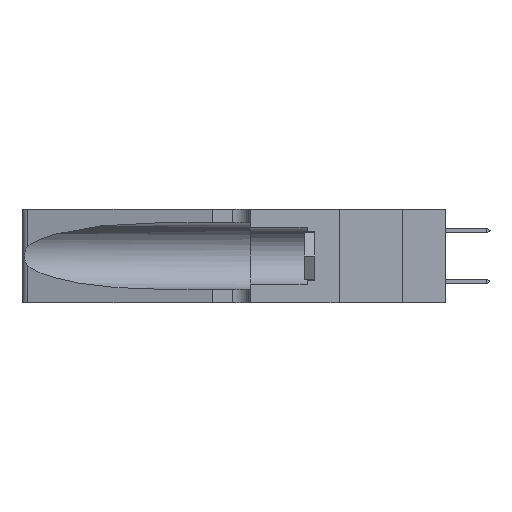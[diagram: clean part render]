
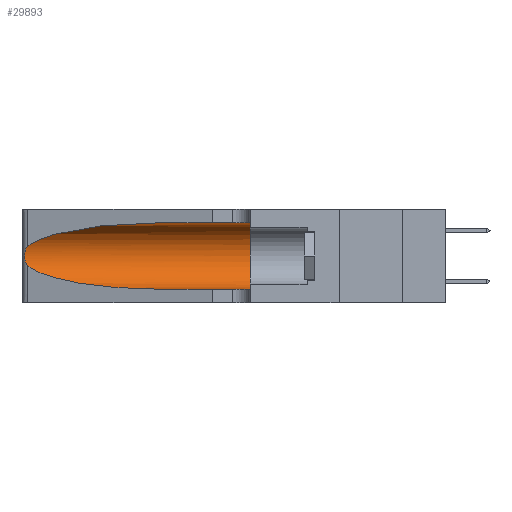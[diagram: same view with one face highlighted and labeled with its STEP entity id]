
A CAD part, left-side view. The second image highlights one B-rep face of the part: STEP entity #29893.
In plain terms, the highlighted cylindrical face has radius 3.308 mm (diameter 6.617 mm), a partial arc.
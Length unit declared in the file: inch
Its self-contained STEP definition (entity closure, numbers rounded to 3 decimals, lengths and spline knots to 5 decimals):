
#35 = DIRECTION ( 'NONE',  ( 0., -1., 0. ) ) ;
#92 = EDGE_CURVE ( 'NONE', #33186, #20749, #12099, .T. ) ;
#208 = ORIENTED_EDGE ( 'NONE', *, *, #2421, .F. ) ;
#2421 = EDGE_CURVE ( 'NONE', #32712, #20749, #4172, .T. ) ;
#4097 = DIRECTION ( 'NONE',  ( 0., -1., 0. ) ) ;
#4172 = CIRCLE ( 'NONE', #7945, 0.13025 ) ;
#4698 = VECTOR ( 'NONE', #35, 39.37008 ) ;
#5731 = EDGE_CURVE ( 'NONE', #13595, #32712, #8255, .T. ) ;
#6392 = CARTESIAN_POINT ( 'NONE',  ( 0.2373, 1.15595, 0.28018 ) ) ;
#7009 = FACE_OUTER_BOUND ( 'NONE', #9619, .T. ) ;
#7945 = AXIS2_PLACEMENT_3D ( 'NONE', #35075, #29318, #26775 ) ;
#8255 = LINE ( 'NONE', #17349, #29503 ) ;
#9052 = CARTESIAN_POINT ( 'NONE',  ( 0.25487, 1.22718, 0.22369 ) ) ;
#9436 = CARTESIAN_POINT ( 'NONE',  ( 0.1305, 1.61858, 0.185 ) ) ;
#9619 = EDGE_LOOP ( 'NONE', ( #25648, #12728, #35269, #34391, #208, #23383 ) ) ;
#9838 = EDGE_CURVE ( 'NONE', #16132, #19628, #12840, .T. ) ;
#10310 = CARTESIAN_POINT ( 'NONE',  ( 0.1305, 0.72297, 0.05475 ) ) ;
#10781 = CARTESIAN_POINT ( 'NONE',  ( 0.25639, 1.23184, 0.21858 ) ) ;
#10813 =( BOUNDED_CURVE ( )  B_SPLINE_CURVE ( 3, ( #31045, #31161, #6392, #9052 ),
 .UNSPECIFIED., .F., .F. ) 
 B_SPLINE_CURVE_WITH_KNOTS ( ( 4, 4 ),
 ( 1.5708, 2.84003 ),
 .UNSPECIFIED. ) 
 CURVE ( )  GEOMETRIC_REPRESENTATION_ITEM ( )  RATIONAL_B_SPLINE_CURVE ( ( 1., 0.87, 0.87, 1. ) ) 
 REPRESENTATION_ITEM ( '' )  );
#11380 = CARTESIAN_POINT ( 'NONE',  ( 0.25856, 1.23593, 0.16098 ) ) ;
#12099 = LINE ( 'NONE', #13935, #4698 ) ;
#12728 = ORIENTED_EDGE ( 'NONE', *, *, #9838, .T. ) ;
#12840 = B_SPLINE_CURVE_WITH_KNOTS ( 'NONE', 3,
 ( #16523, #27407, #10781, #19309, #13617, #16404, #22776, #33714, #16991, #11380, #19875, #22655, #30689, #33484 ),
 .UNSPECIFIED., .F., .F.,
 ( 4, 2, 2, 2, 2, 2, 4 ),
 ( 0., 0.00027, 0.00053, 0.00107, 0.0016, 0.00187, 0.00214 ),
 .UNSPECIFIED. ) ;
#13595 = VERTEX_POINT ( 'NONE', #20034 ) ;
#13617 = CARTESIAN_POINT ( 'NONE',  ( 0.25854, 1.2359, 0.20912 ) ) ;
#13935 = CARTESIAN_POINT ( 'NONE',  ( 0.1305, 1.61858, 0.05475 ) ) ;
#16132 = VERTEX_POINT ( 'NONE', #30842 ) ;
#16357 = CARTESIAN_POINT ( 'NONE',  ( 0.1305, 0.35, 0.05475 ) ) ;
#16404 = CARTESIAN_POINT ( 'NONE',  ( 0.26018, 1.23835, 0.19895 ) ) ;
#16498 = CARTESIAN_POINT ( 'NONE',  ( 0.1305, 0.35, 0.31525 ) ) ;
#16523 = CARTESIAN_POINT ( 'NONE',  ( 0.25487, 1.22718, 0.22369 ) ) ;
#16639 = CYLINDRICAL_SURFACE ( 'NONE', #16894, 0.13025 ) ;
#16894 = AXIS2_PLACEMENT_3D ( 'NONE', #9436, #4097, #28837 ) ;
#16991 = CARTESIAN_POINT ( 'NONE',  ( 0.26017, 1.23833, 0.17102 ) ) ;
#17349 = CARTESIAN_POINT ( 'NONE',  ( 0.1305, 1.61858, 0.31525 ) ) ;
#18951 = CARTESIAN_POINT ( 'NONE',  ( 0.25487, 1.22718, 0.14631 ) ) ;
#19309 = CARTESIAN_POINT ( 'NONE',  ( 0.25787, 1.23484, 0.2124 ) ) ;
#19628 = VERTEX_POINT ( 'NONE', #33997 ) ;
#19875 = CARTESIAN_POINT ( 'NONE',  ( 0.25789, 1.23486, 0.15765 ) ) ;
#20034 = CARTESIAN_POINT ( 'NONE',  ( 0.1305, 0.72297, 0.31525 ) ) ;
#20749 = VERTEX_POINT ( 'NONE', #16357 ) ;
#22655 = CARTESIAN_POINT ( 'NONE',  ( 0.25639, 1.23186, 0.15144 ) ) ;
#22776 = CARTESIAN_POINT ( 'NONE',  ( 0.26075, 1.23896, 0.19203 ) ) ;
#23383 = ORIENTED_EDGE ( 'NONE', *, *, #5731, .F. ) ;
#24248 = CARTESIAN_POINT ( 'NONE',  ( 0.18966, 0.96281, 0.05475 ) ) ;
#25648 = ORIENTED_EDGE ( 'NONE', *, *, #35242, .T. ) ;
#25870 = EDGE_CURVE ( 'NONE', #19628, #33186, #33317, .T. ) ;
#26775 = DIRECTION ( 'NONE',  ( 0., 0., 1. ) ) ;
#27407 = CARTESIAN_POINT ( 'NONE',  ( 0.25555, 1.22994, 0.2215 ) ) ;
#27416 = CARTESIAN_POINT ( 'NONE',  ( 0.2373, 1.15595, 0.08982 ) ) ;
#28837 = DIRECTION ( 'NONE',  ( 0., 0., -1. ) ) ;
#29318 = DIRECTION ( 'NONE',  ( 0., 1., 0. ) ) ;
#29503 = VECTOR ( 'NONE', #35957, 39.37008 ) ;
#29893 = ADVANCED_FACE ( 'NONE', ( #7009 ), #16639, .F. ) ;
#30689 = CARTESIAN_POINT ( 'NONE',  ( 0.25555, 1.22993, 0.14849 ) ) ;
#30842 = CARTESIAN_POINT ( 'NONE',  ( 0.25487, 1.22718, 0.22369 ) ) ;
#31045 = CARTESIAN_POINT ( 'NONE',  ( 0.1305, 0.72297, 0.31525 ) ) ;
#31161 = CARTESIAN_POINT ( 'NONE',  ( 0.18966, 0.96281, 0.31525 ) ) ;
#31481 = CARTESIAN_POINT ( 'NONE',  ( 0.1305, 0.72297, 0.05475 ) ) ;
#32712 = VERTEX_POINT ( 'NONE', #16498 ) ;
#33186 = VERTEX_POINT ( 'NONE', #31481 ) ;
#33317 =( BOUNDED_CURVE ( )  B_SPLINE_CURVE ( 3, ( #18951, #27416, #24248, #10310 ),
 .UNSPECIFIED., .F., .T. ) 
 B_SPLINE_CURVE_WITH_KNOTS ( ( 4, 4 ),
 ( 3.44316, 4.71239 ),
 .UNSPECIFIED. ) 
 CURVE ( )  GEOMETRIC_REPRESENTATION_ITEM ( )  RATIONAL_B_SPLINE_CURVE ( ( 1., 0.87, 0.87, 1. ) ) 
 REPRESENTATION_ITEM ( '' )  );
#33484 = CARTESIAN_POINT ( 'NONE',  ( 0.25487, 1.22718, 0.14631 ) ) ;
#33714 = CARTESIAN_POINT ( 'NONE',  ( 0.26075, 1.23896, 0.178 ) ) ;
#33997 = CARTESIAN_POINT ( 'NONE',  ( 0.25487, 1.22718, 0.14631 ) ) ;
#34391 = ORIENTED_EDGE ( 'NONE', *, *, #92, .T. ) ;
#35075 = CARTESIAN_POINT ( 'NONE',  ( 0.1305, 0.35, 0.185 ) ) ;
#35242 = EDGE_CURVE ( 'NONE', #13595, #16132, #10813, .T. ) ;
#35269 = ORIENTED_EDGE ( 'NONE', *, *, #25870, .T. ) ;
#35957 = DIRECTION ( 'NONE',  ( 0., -1., 0. ) ) ;
